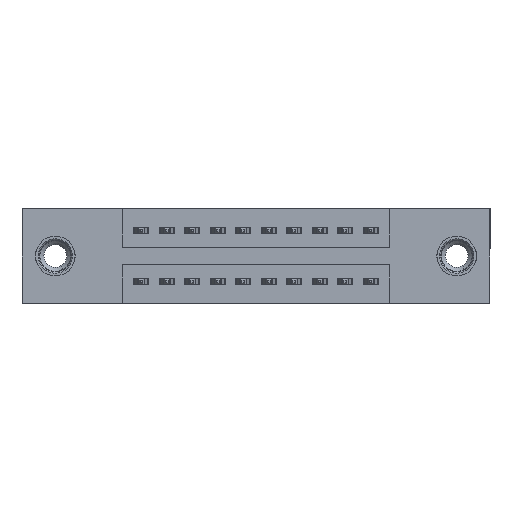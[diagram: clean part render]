
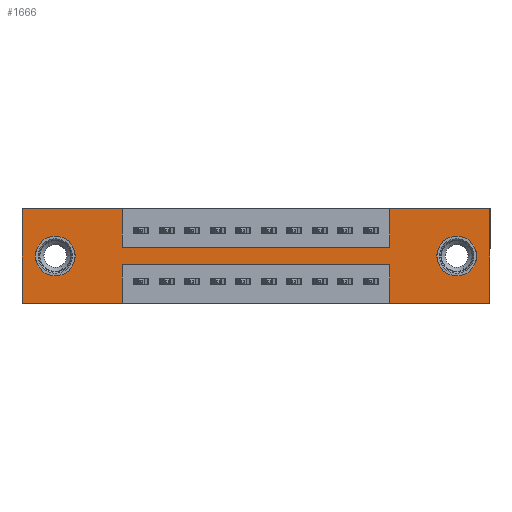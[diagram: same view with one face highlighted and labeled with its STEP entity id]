
A CAD part, front view. The second image highlights one B-rep face of the part: STEP entity #1666.
In plain terms, the highlighted planar face has unit normal (0, -1, 0).
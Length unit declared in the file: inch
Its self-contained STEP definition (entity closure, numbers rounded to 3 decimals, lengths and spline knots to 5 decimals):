
#25 = LINE ( 'NONE', #6198, #5116 ) ;
#101 = CARTESIAN_POINT ( 'NONE',  ( 0.3925, 0., 0. ) ) ;
#227 = ORIENTED_EDGE ( 'NONE', *, *, #1603, .F. ) ;
#413 = DIRECTION ( 'NONE',  ( -1., 0., 0. ) ) ;
#502 = CARTESIAN_POINT ( 'NONE',  ( 1.705, 0., -0.185 ) ) ;
#564 = DIRECTION ( 'NONE',  ( 0., 0., 1. ) ) ;
#670 = VERTEX_POINT ( 'NONE', #4476 ) ;
#699 = LINE ( 'NONE', #1057, #12134 ) ;
#727 = EDGE_CURVE ( 'NONE', #9467, #9730, #5899, .T. ) ;
#818 = ORIENTED_EDGE ( 'NONE', *, *, #13914, .F. ) ;
#886 = VECTOR ( 'NONE', #13521, 39.37008 ) ;
#932 = EDGE_CURVE ( 'NONE', #12014, #3682, #973, .T. ) ;
#973 = LINE ( 'NONE', #2518, #3636 ) ;
#1049 = CARTESIAN_POINT ( 'NONE',  ( 0., 0., 0. ) ) ;
#1057 = CARTESIAN_POINT ( 'NONE',  ( 0.3925, 0., -0.37 ) ) ;
#1316 = AXIS2_PLACEMENT_3D ( 'NONE', #3216, #13240, #10918 ) ;
#1364 = DIRECTION ( 'NONE',  ( 0., 0., -1. ) ) ;
#1437 = CARTESIAN_POINT ( 'NONE',  ( 0.13, 0., -0.185 ) ) ;
#1488 = CARTESIAN_POINT ( 'NONE',  ( 0., 0., -0.37 ) ) ;
#1530 = CARTESIAN_POINT ( 'NONE',  ( 0., 0., -0.37 ) ) ;
#1534 = ORIENTED_EDGE ( 'NONE', *, *, #3485, .F. ) ;
#1603 = EDGE_CURVE ( 'NONE', #6359, #3360, #7784, .T. ) ;
#1629 = CARTESIAN_POINT ( 'NONE',  ( 0., 0., 0. ) ) ;
#1666 = ADVANCED_FACE ( 'NONE', ( #9153, #12933, #4666 ), #2551, .T. ) ;
#1685 = EDGE_CURVE ( 'NONE', #14290, #12071, #5873, .T. ) ;
#1814 = LINE ( 'NONE', #4272, #5167 ) ;
#1922 = ORIENTED_EDGE ( 'NONE', *, *, #932, .F. ) ;
#2395 = CARTESIAN_POINT ( 'NONE',  ( 0.13, 0., -0.107 ) ) ;
#2518 = CARTESIAN_POINT ( 'NONE',  ( 0., 0., -0.37 ) ) ;
#2551 = PLANE ( 'NONE',  #13397 ) ;
#3071 = VERTEX_POINT ( 'NONE', #9432 ) ;
#3204 = EDGE_CURVE ( 'NONE', #12071, #14111, #1814, .T. ) ;
#3216 = CARTESIAN_POINT ( 'NONE',  ( 1.705, 0., -0.185 ) ) ;
#3226 = DIRECTION ( 'NONE',  ( 0., 1., 0. ) ) ;
#3360 = VERTEX_POINT ( 'NONE', #5803 ) ;
#3485 = EDGE_CURVE ( 'NONE', #10809, #14290, #6703, .T. ) ;
#3636 = VECTOR ( 'NONE', #12502, 39.37008 ) ;
#3682 = VERTEX_POINT ( 'NONE', #10707 ) ;
#3868 = DIRECTION ( 'NONE',  ( 0., 0., -1. ) ) ;
#4272 = CARTESIAN_POINT ( 'NONE',  ( 1.835, 0., 0. ) ) ;
#4467 = CIRCLE ( 'NONE', #10045, 0.078 ) ;
#4470 = CARTESIAN_POINT ( 'NONE',  ( 0., 0., 0. ) ) ;
#4476 = CARTESIAN_POINT ( 'NONE',  ( 1.4425, 0., -0.22 ) ) ;
#4547 = CARTESIAN_POINT ( 'NONE',  ( 0.13, 0., -0.185 ) ) ;
#4666 = FACE_OUTER_BOUND ( 'NONE', #6365, .T. ) ;
#4722 = CARTESIAN_POINT ( 'NONE',  ( 0.13, 0., -0.263 ) ) ;
#5040 = ORIENTED_EDGE ( 'NONE', *, *, #12423, .F. ) ;
#5051 = VERTEX_POINT ( 'NONE', #12255 ) ;
#5116 = VECTOR ( 'NONE', #564, 39.37008 ) ;
#5167 = VECTOR ( 'NONE', #7701, 39.37008 ) ;
#5381 = VERTEX_POINT ( 'NONE', #6189 ) ;
#5471 = DIRECTION ( 'NONE',  ( 0., 0., 1. ) ) ;
#5694 = CARTESIAN_POINT ( 'NONE',  ( 1.705, 0., -0.107 ) ) ;
#5759 = CARTESIAN_POINT ( 'NONE',  ( 1.835, 0., -0.37 ) ) ;
#5803 = CARTESIAN_POINT ( 'NONE',  ( 0.3925, 0., -0.15 ) ) ;
#5873 = LINE ( 'NONE', #1629, #9820 ) ;
#5899 = CIRCLE ( 'NONE', #1316, 0.078 ) ;
#5910 = AXIS2_PLACEMENT_3D ( 'NONE', #502, #3226, #1364 ) ;
#5953 = DIRECTION ( 'NONE',  ( 1., 0., 0. ) ) ;
#5988 = LINE ( 'NONE', #8538, #886 ) ;
#6025 = ORIENTED_EDGE ( 'NONE', *, *, #8023, .F. ) ;
#6051 = DIRECTION ( 'NONE',  ( 0., 0., 1. ) ) ;
#6142 = EDGE_LOOP ( 'NONE', ( #13717, #14208 ) ) ;
#6147 = DIRECTION ( 'NONE',  ( 0., -1., 0. ) ) ;
#6189 = CARTESIAN_POINT ( 'NONE',  ( 0., 0., 0. ) ) ;
#6198 = CARTESIAN_POINT ( 'NONE',  ( 1.4425, 0., -0.37 ) ) ;
#6225 = LINE ( 'NONE', #4470, #11021 ) ;
#6359 = VERTEX_POINT ( 'NONE', #101 ) ;
#6365 = EDGE_LOOP ( 'NONE', ( #818, #9066, #5040, #6025, #8640, #12694, #1534, #9564, #227, #10490, #11016, #1922 ) ) ;
#6437 = CARTESIAN_POINT ( 'NONE',  ( 0.3925, 0., -0.37 ) ) ;
#6703 = LINE ( 'NONE', #12643, #12043 ) ;
#6914 = CARTESIAN_POINT ( 'NONE',  ( 0.3925, 0., 0. ) ) ;
#6961 = DIRECTION ( 'NONE',  ( 0., 1., 0. ) ) ;
#7628 = EDGE_LOOP ( 'NONE', ( #12031, #13869 ) ) ;
#7700 = CIRCLE ( 'NONE', #5910, 0.078 ) ;
#7701 = DIRECTION ( 'NONE',  ( 0., 0., -1. ) ) ;
#7709 = VECTOR ( 'NONE', #14089, 39.37008 ) ;
#7736 = EDGE_CURVE ( 'NONE', #13657, #7904, #7881, .T. ) ;
#7784 = LINE ( 'NONE', #6914, #12239 ) ;
#7845 = EDGE_CURVE ( 'NONE', #3360, #10809, #14250, .T. ) ;
#7881 = CIRCLE ( 'NONE', #12820, 0.078 ) ;
#7882 = DIRECTION ( 'NONE',  ( 0., 0., 1. ) ) ;
#7904 = VERTEX_POINT ( 'NONE', #2395 ) ;
#8023 = EDGE_CURVE ( 'NONE', #14111, #5051, #13025, .T. ) ;
#8035 = DIRECTION ( 'NONE',  ( 0., 0., -1. ) ) ;
#8331 = CARTESIAN_POINT ( 'NONE',  ( 1.835, 0., 0. ) ) ;
#8538 = CARTESIAN_POINT ( 'NONE',  ( 0.3925, 0., -0.22 ) ) ;
#8640 = ORIENTED_EDGE ( 'NONE', *, *, #3204, .F. ) ;
#8703 = EDGE_CURVE ( 'NONE', #5381, #6359, #9726, .T. ) ;
#9004 = CARTESIAN_POINT ( 'NONE',  ( 1.4425, 0., -0.15 ) ) ;
#9066 = ORIENTED_EDGE ( 'NONE', *, *, #13267, .F. ) ;
#9153 = FACE_BOUND ( 'NONE', #7628, .T. ) ;
#9432 = CARTESIAN_POINT ( 'NONE',  ( 0.3925, 0., -0.22 ) ) ;
#9467 = VERTEX_POINT ( 'NONE', #5694 ) ;
#9564 = ORIENTED_EDGE ( 'NONE', *, *, #7845, .F. ) ;
#9726 = LINE ( 'NONE', #1049, #13347 ) ;
#9730 = VERTEX_POINT ( 'NONE', #12927 ) ;
#9802 = DIRECTION ( 'NONE',  ( 1., 0., 0. ) ) ;
#9820 = VECTOR ( 'NONE', #5953, 39.37008 ) ;
#10045 = AXIS2_PLACEMENT_3D ( 'NONE', #1437, #6961, #13494 ) ;
#10090 = VECTOR ( 'NONE', #413, 39.37008 ) ;
#10490 = ORIENTED_EDGE ( 'NONE', *, *, #8703, .F. ) ;
#10545 = EDGE_CURVE ( 'NONE', #3682, #5381, #6225, .T. ) ;
#10707 = CARTESIAN_POINT ( 'NONE',  ( 0., 0., -0.37 ) ) ;
#10809 = VERTEX_POINT ( 'NONE', #9004 ) ;
#10827 = EDGE_CURVE ( 'NONE', #7904, #13657, #4467, .T. ) ;
#10918 = DIRECTION ( 'NONE',  ( 0., 0., -1. ) ) ;
#11016 = ORIENTED_EDGE ( 'NONE', *, *, #10545, .F. ) ;
#11021 = VECTOR ( 'NONE', #5471, 39.37008 ) ;
#11410 = DIRECTION ( 'NONE',  ( 0., 0., -1. ) ) ;
#12014 = VERTEX_POINT ( 'NONE', #6437 ) ;
#12031 = ORIENTED_EDGE ( 'NONE', *, *, #727, .T. ) ;
#12043 = VECTOR ( 'NONE', #6051, 39.37008 ) ;
#12071 = VERTEX_POINT ( 'NONE', #8331 ) ;
#12134 = VECTOR ( 'NONE', #11410, 39.37008 ) ;
#12239 = VECTOR ( 'NONE', #8035, 39.37008 ) ;
#12255 = CARTESIAN_POINT ( 'NONE',  ( 1.4425, 0., -0.37 ) ) ;
#12297 = CARTESIAN_POINT ( 'NONE',  ( 0.3925, 0., -0.15 ) ) ;
#12423 = EDGE_CURVE ( 'NONE', #5051, #670, #25, .T. ) ;
#12502 = DIRECTION ( 'NONE',  ( -1., 0., 0. ) ) ;
#12643 = CARTESIAN_POINT ( 'NONE',  ( 1.4425, 0., 0. ) ) ;
#12694 = ORIENTED_EDGE ( 'NONE', *, *, #1685, .F. ) ;
#12820 = AXIS2_PLACEMENT_3D ( 'NONE', #4547, #14186, #7882 ) ;
#12927 = CARTESIAN_POINT ( 'NONE',  ( 1.705, 0., -0.263 ) ) ;
#12933 = FACE_BOUND ( 'NONE', #6142, .T. ) ;
#13025 = LINE ( 'NONE', #1530, #10090 ) ;
#13225 = CARTESIAN_POINT ( 'NONE',  ( 1.4425, 0., 0. ) ) ;
#13240 = DIRECTION ( 'NONE',  ( 0., 1., 0. ) ) ;
#13267 = EDGE_CURVE ( 'NONE', #670, #3071, #5988, .T. ) ;
#13293 = EDGE_CURVE ( 'NONE', #9730, #9467, #7700, .T. ) ;
#13347 = VECTOR ( 'NONE', #9802, 39.37008 ) ;
#13397 = AXIS2_PLACEMENT_3D ( 'NONE', #1488, #6147, #3868 ) ;
#13494 = DIRECTION ( 'NONE',  ( 0., 0., 1. ) ) ;
#13521 = DIRECTION ( 'NONE',  ( -1., 0., 0. ) ) ;
#13657 = VERTEX_POINT ( 'NONE', #4722 ) ;
#13717 = ORIENTED_EDGE ( 'NONE', *, *, #10827, .T. ) ;
#13869 = ORIENTED_EDGE ( 'NONE', *, *, #13293, .T. ) ;
#13914 = EDGE_CURVE ( 'NONE', #3071, #12014, #699, .T. ) ;
#14089 = DIRECTION ( 'NONE',  ( 1., 0., 0. ) ) ;
#14111 = VERTEX_POINT ( 'NONE', #5759 ) ;
#14186 = DIRECTION ( 'NONE',  ( 0., 1., 0. ) ) ;
#14208 = ORIENTED_EDGE ( 'NONE', *, *, #7736, .T. ) ;
#14250 = LINE ( 'NONE', #12297, #7709 ) ;
#14290 = VERTEX_POINT ( 'NONE', #13225 ) ;
